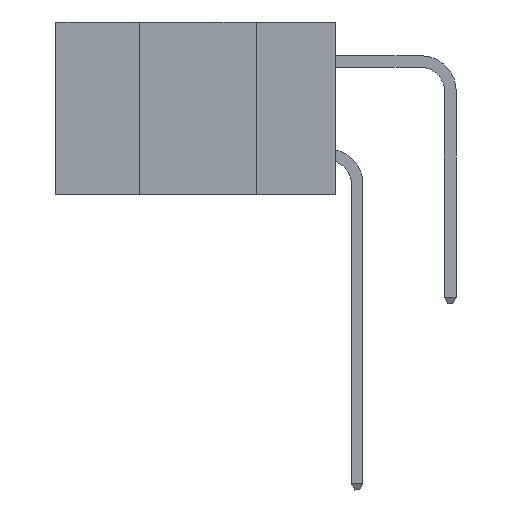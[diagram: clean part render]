
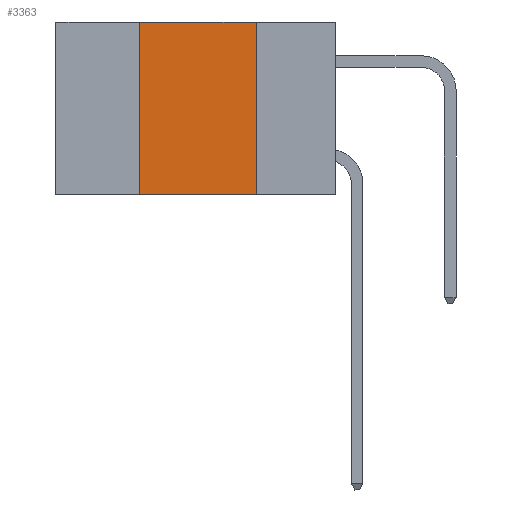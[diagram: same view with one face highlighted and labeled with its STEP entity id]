
A CAD part, left-side view. The second image highlights one B-rep face of the part: STEP entity #3363.
In plain terms, the highlighted planar face has unit normal (-1, 0, 0).
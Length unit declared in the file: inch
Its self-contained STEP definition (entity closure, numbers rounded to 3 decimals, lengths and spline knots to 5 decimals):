
#542 = DIRECTION ( 'NONE',  ( 0., -1., 0. ) ) ;
#945 = VERTEX_POINT ( 'NONE', #24017 ) ;
#996 = CARTESIAN_POINT ( 'NONE',  ( 0., 0.17, 0. ) ) ;
#1514 = VERTEX_POINT ( 'NONE', #27693 ) ;
#1988 = PLANE ( 'NONE',  #21167 ) ;
#3363 = ADVANCED_FACE ( 'NONE', ( #28710 ), #1988, .F. ) ;
#3873 = EDGE_CURVE ( 'NONE', #14809, #19151, #15789, .T. ) ;
#4452 = EDGE_CURVE ( 'NONE', #1514, #14809, #12712, .T. ) ;
#5491 = ORIENTED_EDGE ( 'NONE', *, *, #21552, .T. ) ;
#8556 = CARTESIAN_POINT ( 'NONE',  ( 0., 0.17, 0. ) ) ;
#9646 = CARTESIAN_POINT ( 'NONE',  ( 0., 0.42, 0. ) ) ;
#10209 = VECTOR ( 'NONE', #31228, 39.37008 ) ;
#11253 = ORIENTED_EDGE ( 'NONE', *, *, #3873, .F. ) ;
#11360 = EDGE_CURVE ( 'NONE', #945, #1514, #32242, .T. ) ;
#12062 = EDGE_LOOP ( 'NONE', ( #11253, #24436, #41334, #5491 ) ) ;
#12712 = LINE ( 'NONE', #23382, #17268 ) ;
#14104 = DIRECTION ( 'NONE',  ( 0., -1., 0. ) ) ;
#14809 = VERTEX_POINT ( 'NONE', #996 ) ;
#15207 = LINE ( 'NONE', #26372, #19295 ) ;
#15789 = LINE ( 'NONE', #8556, #10209 ) ;
#17268 = VECTOR ( 'NONE', #14104, 39.37008 ) ;
#19151 = VERTEX_POINT ( 'NONE', #35931 ) ;
#19295 = VECTOR ( 'NONE', #542, 39.37008 ) ;
#21167 = AXIS2_PLACEMENT_3D ( 'NONE', #41755, #24902, #28230 ) ;
#21552 = EDGE_CURVE ( 'NONE', #945, #19151, #15207, .T. ) ;
#23382 = CARTESIAN_POINT ( 'NONE',  ( 0., 0.6, 0. ) ) ;
#24017 = CARTESIAN_POINT ( 'NONE',  ( 0., 0.42, -0.37 ) ) ;
#24436 = ORIENTED_EDGE ( 'NONE', *, *, #4452, .F. ) ;
#24902 = DIRECTION ( 'NONE',  ( 1., 0., 0. ) ) ;
#26372 = CARTESIAN_POINT ( 'NONE',  ( 0., 0.6, -0.37 ) ) ;
#27634 = VECTOR ( 'NONE', #29152, 39.37008 ) ;
#27693 = CARTESIAN_POINT ( 'NONE',  ( 0., 0.42, 0. ) ) ;
#28230 = DIRECTION ( 'NONE',  ( 0., 0., -1. ) ) ;
#28710 = FACE_OUTER_BOUND ( 'NONE', #12062, .T. ) ;
#29152 = DIRECTION ( 'NONE',  ( 0., 0., 1. ) ) ;
#31228 = DIRECTION ( 'NONE',  ( 0., 0., -1. ) ) ;
#32242 = LINE ( 'NONE', #9646, #27634 ) ;
#35931 = CARTESIAN_POINT ( 'NONE',  ( 0., 0.17, -0.37 ) ) ;
#41334 = ORIENTED_EDGE ( 'NONE', *, *, #11360, .F. ) ;
#41755 = CARTESIAN_POINT ( 'NONE',  ( 0., 0.6, 0. ) ) ;
